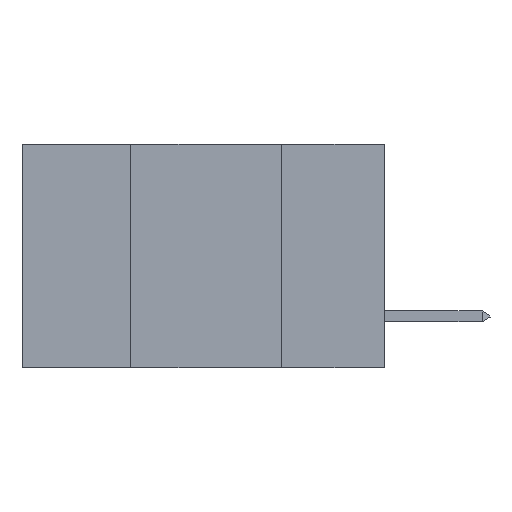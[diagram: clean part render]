
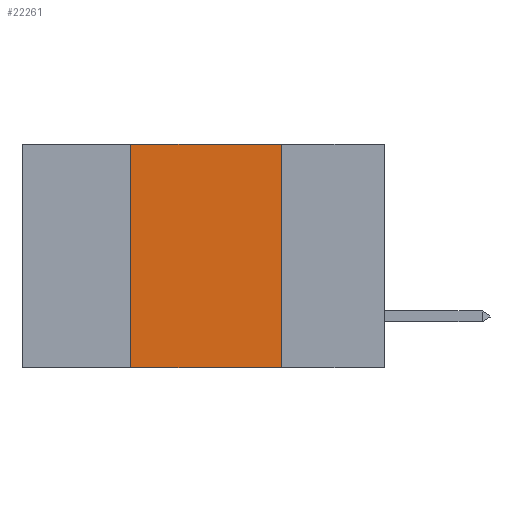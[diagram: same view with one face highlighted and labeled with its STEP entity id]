
A CAD part, left-side view. The second image highlights one B-rep face of the part: STEP entity #22261.
In plain terms, the highlighted planar face has unit normal (-1, 0, 0).
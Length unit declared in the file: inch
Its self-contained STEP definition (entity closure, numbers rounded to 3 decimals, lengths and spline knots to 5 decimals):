
#174 = CARTESIAN_POINT ( 'NONE',  ( 0., 0.17, 0. ) ) ;
#345 = VECTOR ( 'NONE', #2200, 39.37008 ) ;
#761 = EDGE_CURVE ( 'NONE', #12477, #12498, #8967, .T. ) ;
#1979 = PLANE ( 'NONE',  #2010 ) ;
#2010 = AXIS2_PLACEMENT_3D ( 'NONE', #17902, #6027, #19846 ) ;
#2200 = DIRECTION ( 'NONE',  ( 0., -1., 0. ) ) ;
#5668 = ORIENTED_EDGE ( 'NONE', *, *, #761, .F. ) ;
#6027 = DIRECTION ( 'NONE',  ( 1., 0., 0. ) ) ;
#6336 = VERTEX_POINT ( 'NONE', #23578 ) ;
#6397 = CARTESIAN_POINT ( 'NONE',  ( 0., 0.17, -0.37 ) ) ;
#6433 = DIRECTION ( 'NONE',  ( 0., 0., 1. ) ) ;
#6961 = CARTESIAN_POINT ( 'NONE',  ( 0., 0.42, -0.37 ) ) ;
#8889 = EDGE_CURVE ( 'NONE', #6336, #12477, #16298, .T. ) ;
#8967 = LINE ( 'NONE', #10242, #18847 ) ;
#9884 = VECTOR ( 'NONE', #18113, 39.37008 ) ;
#10242 = CARTESIAN_POINT ( 'NONE',  ( 0., 0.17, 0. ) ) ;
#10373 = VERTEX_POINT ( 'NONE', #6961 ) ;
#12028 = LINE ( 'NONE', #16383, #21835 ) ;
#12201 = CARTESIAN_POINT ( 'NONE',  ( 0., 0.6, -0.37 ) ) ;
#12267 = DIRECTION ( 'NONE',  ( 0., 0., -1. ) ) ;
#12477 = VERTEX_POINT ( 'NONE', #174 ) ;
#12498 = VERTEX_POINT ( 'NONE', #6397 ) ;
#13707 = EDGE_CURVE ( 'NONE', #10373, #12498, #25523, .T. ) ;
#14542 = ORIENTED_EDGE ( 'NONE', *, *, #13707, .T. ) ;
#16298 = LINE ( 'NONE', #23901, #345 ) ;
#16383 = CARTESIAN_POINT ( 'NONE',  ( 0., 0.42, 0. ) ) ;
#17902 = CARTESIAN_POINT ( 'NONE',  ( 0., 0.6, 0. ) ) ;
#18113 = DIRECTION ( 'NONE',  ( 0., -1., 0. ) ) ;
#18847 = VECTOR ( 'NONE', #12267, 39.37008 ) ;
#19846 = DIRECTION ( 'NONE',  ( 0., 0., -1. ) ) ;
#21107 = EDGE_CURVE ( 'NONE', #10373, #6336, #12028, .T. ) ;
#21835 = VECTOR ( 'NONE', #6433, 39.37008 ) ;
#22261 = ADVANCED_FACE ( 'NONE', ( #24781 ), #1979, .F. ) ;
#23578 = CARTESIAN_POINT ( 'NONE',  ( 0., 0.42, 0. ) ) ;
#23901 = CARTESIAN_POINT ( 'NONE',  ( 0., 0.6, 0. ) ) ;
#24111 = ORIENTED_EDGE ( 'NONE', *, *, #8889, .F. ) ;
#24781 = FACE_OUTER_BOUND ( 'NONE', #25444, .T. ) ;
#25444 = EDGE_LOOP ( 'NONE', ( #5668, #24111, #25540, #14542 ) ) ;
#25523 = LINE ( 'NONE', #12201, #9884 ) ;
#25540 = ORIENTED_EDGE ( 'NONE', *, *, #21107, .F. ) ;
